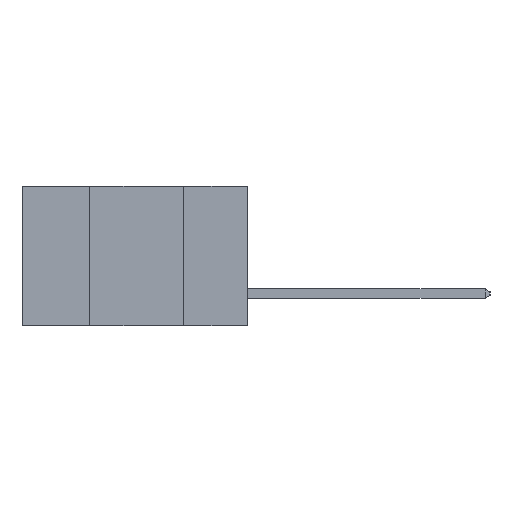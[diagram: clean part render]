
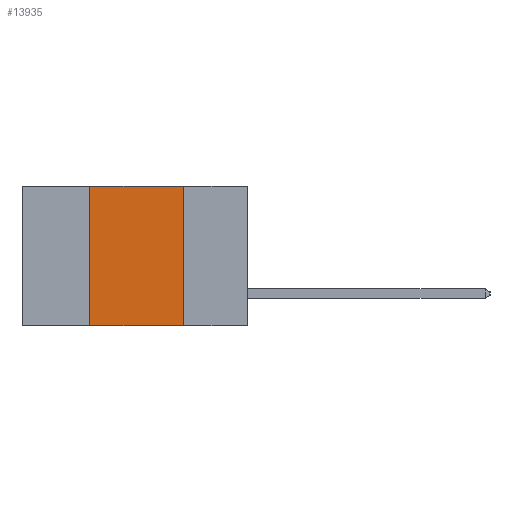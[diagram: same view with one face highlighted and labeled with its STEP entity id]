
A CAD part, left-side view. The second image highlights one B-rep face of the part: STEP entity #13935.
In plain terms, the highlighted planar face has unit normal (-1, 0, 0).
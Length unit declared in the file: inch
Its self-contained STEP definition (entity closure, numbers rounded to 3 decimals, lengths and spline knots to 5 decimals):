
#1795 = VERTEX_POINT ( 'NONE', #17200 ) ;
#2443 = VECTOR ( 'NONE', #19481, 39.37008 ) ;
#2464 = CARTESIAN_POINT ( 'NONE',  ( 0., 0.17, 0. ) ) ;
#2473 = VERTEX_POINT ( 'NONE', #23138 ) ;
#2902 = CARTESIAN_POINT ( 'NONE',  ( 0., 0.42, 0. ) ) ;
#3198 = CARTESIAN_POINT ( 'NONE',  ( 0., 0.17, -0.37 ) ) ;
#3383 = CARTESIAN_POINT ( 'NONE',  ( 0., 0.42, -0.37 ) ) ;
#4283 = EDGE_CURVE ( 'NONE', #5623, #2473, #22017, .T. ) ;
#4892 = AXIS2_PLACEMENT_3D ( 'NONE', #10330, #23939, #12299 ) ;
#5623 = VERTEX_POINT ( 'NONE', #3383 ) ;
#6411 = FACE_OUTER_BOUND ( 'NONE', #18006, .T. ) ;
#7604 = VECTOR ( 'NONE', #11313, 39.37008 ) ;
#10251 = VECTOR ( 'NONE', #20259, 39.37008 ) ;
#10330 = CARTESIAN_POINT ( 'NONE',  ( 0., 0.6, 0. ) ) ;
#10861 = LINE ( 'NONE', #18329, #10251 ) ;
#11313 = DIRECTION ( 'NONE',  ( 0., -1., 0. ) ) ;
#12299 = DIRECTION ( 'NONE',  ( 0., 0., -1. ) ) ;
#13935 = ADVANCED_FACE ( 'NONE', ( #6411 ), #18202, .F. ) ;
#14954 = EDGE_CURVE ( 'NONE', #2473, #1795, #23198, .T. ) ;
#16078 = ORIENTED_EDGE ( 'NONE', *, *, #20539, .F. ) ;
#16552 = ORIENTED_EDGE ( 'NONE', *, *, #4283, .F. ) ;
#17042 = ORIENTED_EDGE ( 'NONE', *, *, #14954, .F. ) ;
#17200 = CARTESIAN_POINT ( 'NONE',  ( 0., 0.17, 0. ) ) ;
#17354 = LINE ( 'NONE', #2464, #21862 ) ;
#17459 = EDGE_CURVE ( 'NONE', #5623, #23153, #10861, .T. ) ;
#18006 = EDGE_LOOP ( 'NONE', ( #16078, #17042, #16552, #21847 ) ) ;
#18195 = DIRECTION ( 'NONE',  ( 0., 0., -1. ) ) ;
#18202 = PLANE ( 'NONE',  #4892 ) ;
#18329 = CARTESIAN_POINT ( 'NONE',  ( 0., 0.6, -0.37 ) ) ;
#19169 = CARTESIAN_POINT ( 'NONE',  ( 0., 0.6, 0. ) ) ;
#19481 = DIRECTION ( 'NONE',  ( 0., 0., 1. ) ) ;
#20259 = DIRECTION ( 'NONE',  ( 0., -1., 0. ) ) ;
#20539 = EDGE_CURVE ( 'NONE', #1795, #23153, #17354, .T. ) ;
#21847 = ORIENTED_EDGE ( 'NONE', *, *, #17459, .T. ) ;
#21862 = VECTOR ( 'NONE', #18195, 39.37008 ) ;
#22017 = LINE ( 'NONE', #2902, #2443 ) ;
#23138 = CARTESIAN_POINT ( 'NONE',  ( 0., 0.42, 0. ) ) ;
#23153 = VERTEX_POINT ( 'NONE', #3198 ) ;
#23198 = LINE ( 'NONE', #19169, #7604 ) ;
#23939 = DIRECTION ( 'NONE',  ( 1., 0., 0. ) ) ;
